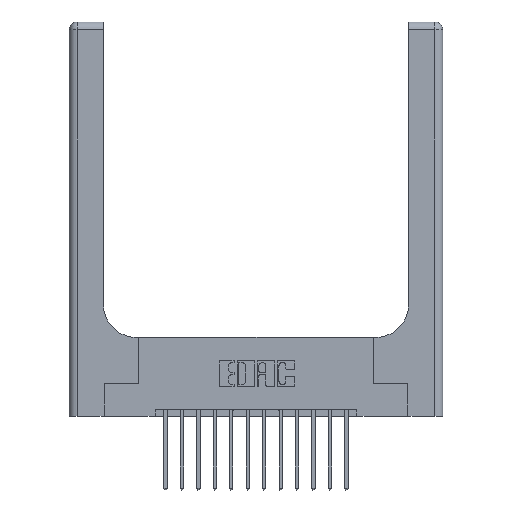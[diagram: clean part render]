
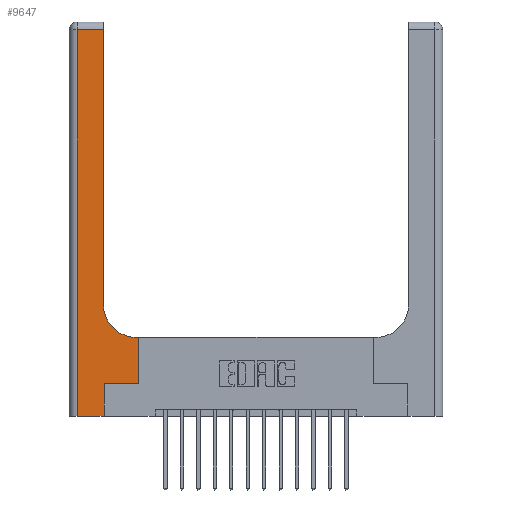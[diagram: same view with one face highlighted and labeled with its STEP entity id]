
A CAD part, top view. The second image highlights one B-rep face of the part: STEP entity #9647.
In plain terms, the highlighted planar face has unit normal (0, 0, 1).
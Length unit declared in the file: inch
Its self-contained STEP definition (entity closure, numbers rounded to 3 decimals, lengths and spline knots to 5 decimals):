
#36 = CARTESIAN_POINT ( 'NONE',  ( 0.528, 0.6, 0.37 ) ) ;
#38 = CARTESIAN_POINT ( 'NONE',  ( 0., 2.94, 0.37 ) ) ;
#475 = VECTOR ( 'NONE', #2830, 39.37008 ) ;
#639 = CARTESIAN_POINT ( 'NONE',  ( 0., 0., 0.37 ) ) ;
#843 = AXIS2_PLACEMENT_3D ( 'NONE', #7633, #11690, #17021 ) ;
#1121 = CARTESIAN_POINT ( 'NONE',  ( 0.26, 0.85, 0.37 ) ) ;
#1205 = CARTESIAN_POINT ( 'NONE',  ( 0.265, 0., 0.37 ) ) ;
#1288 = CARTESIAN_POINT ( 'NONE',  ( 0.26, 2.94, 0.37 ) ) ;
#1362 = LINE ( 'NONE', #38, #7378 ) ;
#1767 = ORIENTED_EDGE ( 'NONE', *, *, #4255, .T. ) ;
#1965 = DIRECTION ( 'NONE',  ( 1., 0., 0. ) ) ;
#2111 = VECTOR ( 'NONE', #10272, 39.37008 ) ;
#2131 = EDGE_CURVE ( 'NONE', #10823, #14553, #7279, .T. ) ;
#2382 = VERTEX_POINT ( 'NONE', #1121 ) ;
#2465 = EDGE_CURVE ( 'NONE', #14553, #17025, #12985, .T. ) ;
#2520 = VERTEX_POINT ( 'NONE', #1288 ) ;
#2830 = DIRECTION ( 'NONE',  ( 0., -1., 0. ) ) ;
#3397 = EDGE_CURVE ( 'NONE', #9082, #2382, #8477, .T. ) ;
#3496 = EDGE_LOOP ( 'NONE', ( #6869, #1767, #14605, #16491, #12384, #11794, #5570, #14854, #12826 ) ) ;
#3978 = CARTESIAN_POINT ( 'NONE',  ( 0.06, 3., 0.37 ) ) ;
#4255 = EDGE_CURVE ( 'NONE', #2520, #17034, #1362, .T. ) ;
#4548 = DIRECTION ( 'NONE',  ( 0., 0., -1. ) ) ;
#5043 = VECTOR ( 'NONE', #1965, 39.37008 ) ;
#5542 = CARTESIAN_POINT ( 'NONE',  ( 0.51, 0.6, 0.37 ) ) ;
#5570 = ORIENTED_EDGE ( 'NONE', *, *, #2465, .T. ) ;
#5786 = CARTESIAN_POINT ( 'NONE',  ( 0.528, 0.25, 0.37 ) ) ;
#6091 = DIRECTION ( 'NONE',  ( 0., 1., 0. ) ) ;
#6349 = VECTOR ( 'NONE', #9764, 39.37008 ) ;
#6815 = LINE ( 'NONE', #3978, #475 ) ;
#6869 = ORIENTED_EDGE ( 'NONE', *, *, #9596, .T. ) ;
#6946 = LINE ( 'NONE', #11012, #6349 ) ;
#7209 = FACE_OUTER_BOUND ( 'NONE', #3496, .T. ) ;
#7246 = EDGE_CURVE ( 'NONE', #14336, #10823, #14172, .T. ) ;
#7279 = LINE ( 'NONE', #14100, #5043 ) ;
#7378 = VECTOR ( 'NONE', #8349, 39.37008 ) ;
#7493 = VECTOR ( 'NONE', #15471, 39.37008 ) ;
#7633 = CARTESIAN_POINT ( 'NONE',  ( 0.51, 0.85, 0.37 ) ) ;
#8349 = DIRECTION ( 'NONE',  ( -1., 0., 0. ) ) ;
#8477 = CIRCLE ( 'NONE', #843, 0.25 ) ;
#9082 = VERTEX_POINT ( 'NONE', #5542 ) ;
#9088 = DIRECTION ( 'NONE',  ( 0., 1., 0. ) ) ;
#9596 = EDGE_CURVE ( 'NONE', #2382, #2520, #6946, .T. ) ;
#9647 = ADVANCED_FACE ( 'NONE', ( #7209 ), #12595, .F. ) ;
#9763 = EDGE_CURVE ( 'NONE', #14072, #14336, #11696, .T. ) ;
#9764 = DIRECTION ( 'NONE',  ( 0., 1., 0. ) ) ;
#9933 = DIRECTION ( 'NONE',  ( -1., 0., 0. ) ) ;
#10272 = DIRECTION ( 'NONE',  ( 1., 0., 0. ) ) ;
#10429 = VECTOR ( 'NONE', #9088, 39.37008 ) ;
#10823 = VERTEX_POINT ( 'NONE', #13016 ) ;
#11012 = CARTESIAN_POINT ( 'NONE',  ( 0.26, 3., 0.37 ) ) ;
#11460 = LINE ( 'NONE', #11725, #7493 ) ;
#11690 = DIRECTION ( 'NONE',  ( 0., 0., -1. ) ) ;
#11696 = LINE ( 'NONE', #639, #2111 ) ;
#11725 = CARTESIAN_POINT ( 'NONE',  ( 0.26, 0.6, 0.37 ) ) ;
#11794 = ORIENTED_EDGE ( 'NONE', *, *, #2131, .T. ) ;
#11924 = CARTESIAN_POINT ( 'NONE',  ( 0.528, 0.25, 0.37 ) ) ;
#12384 = ORIENTED_EDGE ( 'NONE', *, *, #7246, .T. ) ;
#12595 = PLANE ( 'NONE',  #15135 ) ;
#12826 = ORIENTED_EDGE ( 'NONE', *, *, #3397, .T. ) ;
#12827 = CARTESIAN_POINT ( 'NONE',  ( 0.265, 0., 0.37 ) ) ;
#12985 = LINE ( 'NONE', #11924, #10429 ) ;
#13016 = CARTESIAN_POINT ( 'NONE',  ( 0.265, 0.25, 0.37 ) ) ;
#14072 = VERTEX_POINT ( 'NONE', #14979 ) ;
#14100 = CARTESIAN_POINT ( 'NONE',  ( 0.265, 0.25, 0.37 ) ) ;
#14172 = LINE ( 'NONE', #12827, #16080 ) ;
#14302 = EDGE_CURVE ( 'NONE', #17025, #9082, #11460, .T. ) ;
#14336 = VERTEX_POINT ( 'NONE', #1205 ) ;
#14553 = VERTEX_POINT ( 'NONE', #5786 ) ;
#14605 = ORIENTED_EDGE ( 'NONE', *, *, #15299, .T. ) ;
#14749 = CARTESIAN_POINT ( 'NONE',  ( 0.06, 2.94, 0.37 ) ) ;
#14854 = ORIENTED_EDGE ( 'NONE', *, *, #14302, .T. ) ;
#14979 = CARTESIAN_POINT ( 'NONE',  ( 0.06, 0., 0.37 ) ) ;
#15135 = AXIS2_PLACEMENT_3D ( 'NONE', #16690, #4548, #9933 ) ;
#15299 = EDGE_CURVE ( 'NONE', #17034, #14072, #6815, .T. ) ;
#15471 = DIRECTION ( 'NONE',  ( -1., 0., 0. ) ) ;
#16080 = VECTOR ( 'NONE', #6091, 39.37008 ) ;
#16491 = ORIENTED_EDGE ( 'NONE', *, *, #9763, .T. ) ;
#16690 = CARTESIAN_POINT ( 'NONE',  ( 0., 3., 0.37 ) ) ;
#17021 = DIRECTION ( 'NONE',  ( 1., 0., 0. ) ) ;
#17025 = VERTEX_POINT ( 'NONE', #36 ) ;
#17034 = VERTEX_POINT ( 'NONE', #14749 ) ;
